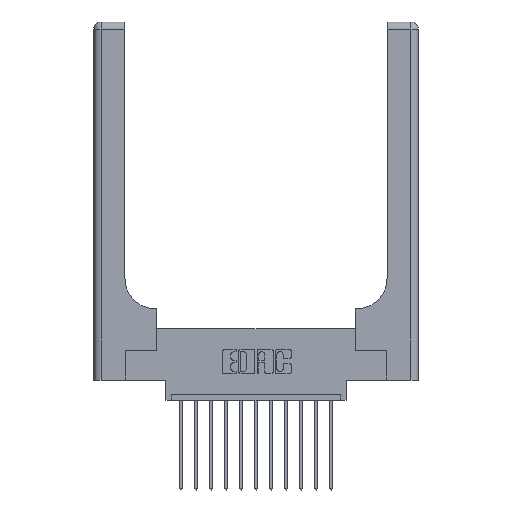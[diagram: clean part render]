
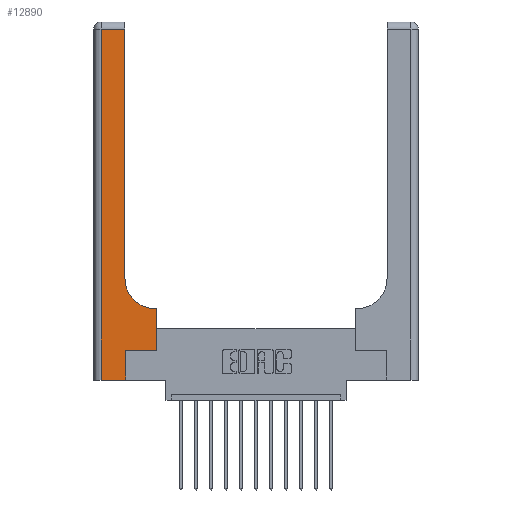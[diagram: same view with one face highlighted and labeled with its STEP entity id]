
A CAD part, top view. The second image highlights one B-rep face of the part: STEP entity #12890.
In plain terms, the highlighted planar face has unit normal (0, 0, 1).
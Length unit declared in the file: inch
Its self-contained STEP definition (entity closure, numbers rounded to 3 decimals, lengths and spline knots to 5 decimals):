
#50 = LINE ( 'NONE', #11485, #9005 ) ;
#225 = ORIENTED_EDGE ( 'NONE', *, *, #6968, .T. ) ;
#229 = DIRECTION ( 'NONE',  ( 0., 0., -1. ) ) ;
#567 = LINE ( 'NONE', #903, #13537 ) ;
#574 = CARTESIAN_POINT ( 'NONE',  ( 0.265, 0., 0.37 ) ) ;
#903 = CARTESIAN_POINT ( 'NONE',  ( 0.528, 0.25, 0.37 ) ) ;
#1120 = ORIENTED_EDGE ( 'NONE', *, *, #3196, .T. ) ;
#1673 = EDGE_LOOP ( 'NONE', ( #12715, #1120, #225, #3276, #3811, #2077, #14072, #16371, #8729 ) ) ;
#2077 = ORIENTED_EDGE ( 'NONE', *, *, #8836, .T. ) ;
#2604 = DIRECTION ( 'NONE',  ( 0., 1., 0. ) ) ;
#2818 = CARTESIAN_POINT ( 'NONE',  ( 0.51, 0.85, 0.37 ) ) ;
#2914 = CARTESIAN_POINT ( 'NONE',  ( 0., 3., 0.37 ) ) ;
#3196 = EDGE_CURVE ( 'NONE', #5715, #3397, #7283, .T. ) ;
#3276 = ORIENTED_EDGE ( 'NONE', *, *, #11932, .T. ) ;
#3397 = VERTEX_POINT ( 'NONE', #5176 ) ;
#3811 = ORIENTED_EDGE ( 'NONE', *, *, #16549, .T. ) ;
#4200 = LINE ( 'NONE', #9376, #16134 ) ;
#4746 = CARTESIAN_POINT ( 'NONE',  ( 0.26, 0.6, 0.37 ) ) ;
#4837 = DIRECTION ( 'NONE',  ( -1., 0., 0. ) ) ;
#5151 = DIRECTION ( 'NONE',  ( 1., 0., 0. ) ) ;
#5176 = CARTESIAN_POINT ( 'NONE',  ( 0.06, 2.94, 0.37 ) ) ;
#5504 = CARTESIAN_POINT ( 'NONE',  ( 0.265, 0., 0.37 ) ) ;
#5715 = VERTEX_POINT ( 'NONE', #11092 ) ;
#5772 = CARTESIAN_POINT ( 'NONE',  ( 0., 2.94, 0.37 ) ) ;
#5850 = DIRECTION ( 'NONE',  ( 0., 1., 0. ) ) ;
#5858 = EDGE_CURVE ( 'NONE', #13535, #10458, #567, .T. ) ;
#5924 = CARTESIAN_POINT ( 'NONE',  ( 0.26, 0.85, 0.37 ) ) ;
#6705 = DIRECTION ( 'NONE',  ( 1., 0., 0. ) ) ;
#6968 = EDGE_CURVE ( 'NONE', #3397, #12776, #50, .T. ) ;
#7040 = VERTEX_POINT ( 'NONE', #9073 ) ;
#7283 = LINE ( 'NONE', #5772, #10828 ) ;
#7558 = DIRECTION ( 'NONE',  ( 0., -1., 0. ) ) ;
#7953 = CARTESIAN_POINT ( 'NONE',  ( 0., 0., 0.37 ) ) ;
#7985 = DIRECTION ( 'NONE',  ( 0., 0., -1. ) ) ;
#8031 = LINE ( 'NONE', #7953, #12828 ) ;
#8079 = FACE_OUTER_BOUND ( 'NONE', #1673, .T. ) ;
#8402 = LINE ( 'NONE', #4746, #12177 ) ;
#8729 = ORIENTED_EDGE ( 'NONE', *, *, #14240, .T. ) ;
#8836 = EDGE_CURVE ( 'NONE', #7040, #13535, #8958, .T. ) ;
#8958 = LINE ( 'NONE', #12723, #8997 ) ;
#8997 = VECTOR ( 'NONE', #5151, 39.37008 ) ;
#9005 = VECTOR ( 'NONE', #7558, 39.37008 ) ;
#9037 = LINE ( 'NONE', #574, #10475 ) ;
#9073 = CARTESIAN_POINT ( 'NONE',  ( 0.265, 0.25, 0.37 ) ) ;
#9376 = CARTESIAN_POINT ( 'NONE',  ( 0.26, 3., 0.37 ) ) ;
#9600 = DIRECTION ( 'NONE',  ( -1., 0., 0. ) ) ;
#9906 = AXIS2_PLACEMENT_3D ( 'NONE', #2818, #7985, #6705 ) ;
#10458 = VERTEX_POINT ( 'NONE', #11891 ) ;
#10475 = VECTOR ( 'NONE', #2604, 39.37008 ) ;
#10591 = VERTEX_POINT ( 'NONE', #5924 ) ;
#10828 = VECTOR ( 'NONE', #9600, 39.37008 ) ;
#11092 = CARTESIAN_POINT ( 'NONE',  ( 0.26, 2.94, 0.37 ) ) ;
#11349 = EDGE_CURVE ( 'NONE', #10458, #11803, #8402, .T. ) ;
#11485 = CARTESIAN_POINT ( 'NONE',  ( 0.06, 3., 0.37 ) ) ;
#11531 = VERTEX_POINT ( 'NONE', #5504 ) ;
#11757 = DIRECTION ( 'NONE',  ( -1., 0., 0. ) ) ;
#11803 = VERTEX_POINT ( 'NONE', #15097 ) ;
#11891 = CARTESIAN_POINT ( 'NONE',  ( 0.528, 0.6, 0.37 ) ) ;
#11932 = EDGE_CURVE ( 'NONE', #12776, #11531, #8031, .T. ) ;
#12128 = DIRECTION ( 'NONE',  ( 1., 0., 0. ) ) ;
#12177 = VECTOR ( 'NONE', #4837, 39.37008 ) ;
#12326 = EDGE_CURVE ( 'NONE', #10591, #5715, #4200, .T. ) ;
#12715 = ORIENTED_EDGE ( 'NONE', *, *, #12326, .T. ) ;
#12723 = CARTESIAN_POINT ( 'NONE',  ( 0.265, 0.25, 0.37 ) ) ;
#12776 = VERTEX_POINT ( 'NONE', #13028 ) ;
#12828 = VECTOR ( 'NONE', #12128, 39.37008 ) ;
#12890 = ADVANCED_FACE ( 'NONE', ( #8079 ), #14538, .F. ) ;
#13028 = CARTESIAN_POINT ( 'NONE',  ( 0.06, 0., 0.37 ) ) ;
#13417 = CIRCLE ( 'NONE', #9906, 0.25 ) ;
#13535 = VERTEX_POINT ( 'NONE', #15496 ) ;
#13537 = VECTOR ( 'NONE', #5850, 39.37008 ) ;
#14072 = ORIENTED_EDGE ( 'NONE', *, *, #5858, .T. ) ;
#14240 = EDGE_CURVE ( 'NONE', #11803, #10591, #13417, .T. ) ;
#14538 = PLANE ( 'NONE',  #16213 ) ;
#14560 = DIRECTION ( 'NONE',  ( 0., 1., 0. ) ) ;
#15097 = CARTESIAN_POINT ( 'NONE',  ( 0.51, 0.6, 0.37 ) ) ;
#15496 = CARTESIAN_POINT ( 'NONE',  ( 0.528, 0.25, 0.37 ) ) ;
#16134 = VECTOR ( 'NONE', #14560, 39.37008 ) ;
#16213 = AXIS2_PLACEMENT_3D ( 'NONE', #2914, #229, #11757 ) ;
#16371 = ORIENTED_EDGE ( 'NONE', *, *, #11349, .T. ) ;
#16549 = EDGE_CURVE ( 'NONE', #11531, #7040, #9037, .T. ) ;
